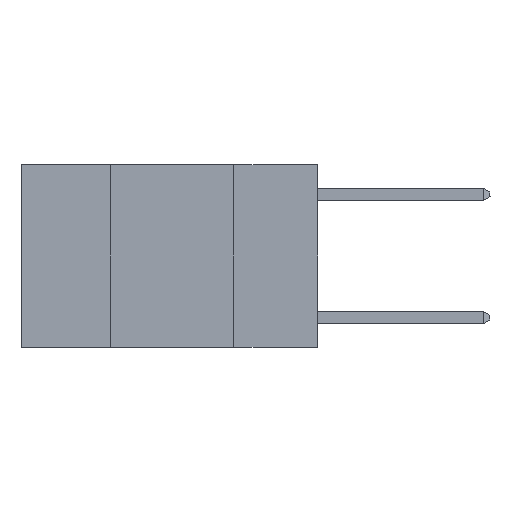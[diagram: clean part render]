
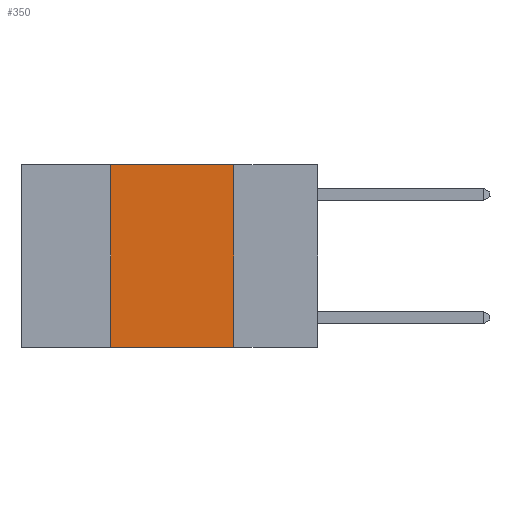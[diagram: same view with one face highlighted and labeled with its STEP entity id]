
A CAD part, left-side view. The second image highlights one B-rep face of the part: STEP entity #350.
In plain terms, the highlighted planar face has unit normal (-1, 0, 0).
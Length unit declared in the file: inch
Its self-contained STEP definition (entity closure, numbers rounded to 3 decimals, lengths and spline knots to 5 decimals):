
#239 = ORIENTED_EDGE ( 'NONE', *, *, #5357, .T. ) ;
#350 = ADVANCED_FACE ( 'NONE', ( #2127 ), #9968, .F. ) ;
#374 = ORIENTED_EDGE ( 'NONE', *, *, #9451, .F. ) ;
#402 = DIRECTION ( 'NONE',  ( 1., 0., 0. ) ) ;
#452 = VECTOR ( 'NONE', #3817, 39.37008 ) ;
#471 = DIRECTION ( 'NONE',  ( 0., 0., -1. ) ) ;
#1421 = LINE ( 'NONE', #3254, #5043 ) ;
#2127 = FACE_OUTER_BOUND ( 'NONE', #11137, .T. ) ;
#2742 = ORIENTED_EDGE ( 'NONE', *, *, #11726, .F. ) ;
#3045 = CARTESIAN_POINT ( 'NONE',  ( 0., 0.42, 0. ) ) ;
#3254 = CARTESIAN_POINT ( 'NONE',  ( 0., 0.42, 0. ) ) ;
#3578 = VECTOR ( 'NONE', #471, 39.37008 ) ;
#3693 = AXIS2_PLACEMENT_3D ( 'NONE', #9006, #402, #5947 ) ;
#3817 = DIRECTION ( 'NONE',  ( 0., -1., 0. ) ) ;
#4446 = LINE ( 'NONE', #8127, #3578 ) ;
#4706 = ORIENTED_EDGE ( 'NONE', *, *, #5897, .F. ) ;
#5026 = DIRECTION ( 'NONE',  ( 0., 0., 1. ) ) ;
#5043 = VECTOR ( 'NONE', #5026, 39.37008 ) ;
#5357 = EDGE_CURVE ( 'NONE', #8955, #11747, #8900, .T. ) ;
#5897 = EDGE_CURVE ( 'NONE', #9555, #11747, #4446, .T. ) ;
#5947 = DIRECTION ( 'NONE',  ( 0., 0., -1. ) ) ;
#6061 = CARTESIAN_POINT ( 'NONE',  ( 0., 0.17, 0. ) ) ;
#7042 = CARTESIAN_POINT ( 'NONE',  ( 0., 0.6, -0.37 ) ) ;
#8127 = CARTESIAN_POINT ( 'NONE',  ( 0., 0.17, 0. ) ) ;
#8570 = CARTESIAN_POINT ( 'NONE',  ( 0., 0.6, 0. ) ) ;
#8900 = LINE ( 'NONE', #7042, #10396 ) ;
#8955 = VERTEX_POINT ( 'NONE', #11500 ) ;
#9006 = CARTESIAN_POINT ( 'NONE',  ( 0., 0.6, 0. ) ) ;
#9451 = EDGE_CURVE ( 'NONE', #10951, #9555, #10413, .T. ) ;
#9555 = VERTEX_POINT ( 'NONE', #6061 ) ;
#9854 = CARTESIAN_POINT ( 'NONE',  ( 0., 0.17, -0.37 ) ) ;
#9968 = PLANE ( 'NONE',  #3693 ) ;
#10396 = VECTOR ( 'NONE', #10852, 39.37008 ) ;
#10413 = LINE ( 'NONE', #8570, #452 ) ;
#10852 = DIRECTION ( 'NONE',  ( 0., -1., 0. ) ) ;
#10951 = VERTEX_POINT ( 'NONE', #3045 ) ;
#11137 = EDGE_LOOP ( 'NONE', ( #4706, #374, #2742, #239 ) ) ;
#11500 = CARTESIAN_POINT ( 'NONE',  ( 0., 0.42, -0.37 ) ) ;
#11726 = EDGE_CURVE ( 'NONE', #8955, #10951, #1421, .T. ) ;
#11747 = VERTEX_POINT ( 'NONE', #9854 ) ;
